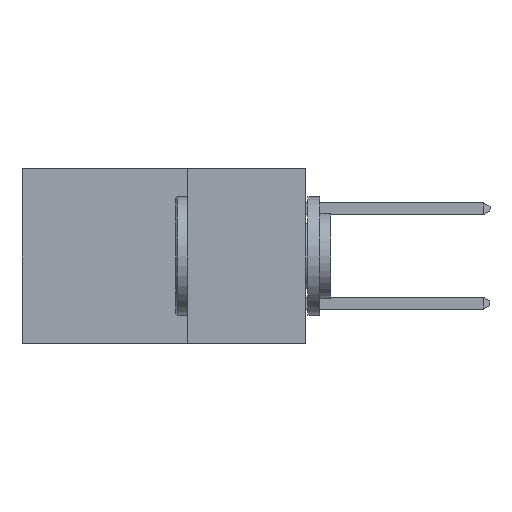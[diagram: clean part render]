
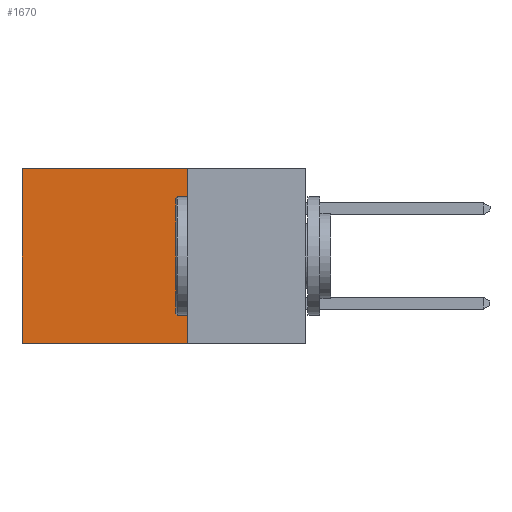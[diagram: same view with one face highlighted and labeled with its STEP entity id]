
A CAD part, left-side view. The second image highlights one B-rep face of the part: STEP entity #1670.
In plain terms, the highlighted planar face has unit normal (-1, 0, 0).
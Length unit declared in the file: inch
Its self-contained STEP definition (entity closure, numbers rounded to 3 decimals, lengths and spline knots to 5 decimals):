
#51 = CARTESIAN_POINT ( 'NONE',  ( 0.2615, 0.25, -0.37 ) ) ;
#232 = VERTEX_POINT ( 'NONE', #9290 ) ;
#253 = VERTEX_POINT ( 'NONE', #899 ) ;
#372 = ORIENTED_EDGE ( 'NONE', *, *, #7196, .F. ) ;
#837 = DIRECTION ( 'NONE',  ( 0., 0., -1. ) ) ;
#899 = CARTESIAN_POINT ( 'NONE',  ( 0.2615, 0.6, -0.37 ) ) ;
#1422 = CARTESIAN_POINT ( 'NONE',  ( 0.2615, 0.25, -0.37 ) ) ;
#1670 = ADVANCED_FACE ( 'NONE', ( #6097 ), #6054, .F. ) ;
#2181 = VECTOR ( 'NONE', #4646, 39.37008 ) ;
#2229 = CARTESIAN_POINT ( 'NONE',  ( 0.2615, 0.25, 0. ) ) ;
#2306 = DIRECTION ( 'NONE',  ( 0., 1., 0. ) ) ;
#3445 = VECTOR ( 'NONE', #7280, 39.37008 ) ;
#3839 = LINE ( 'NONE', #51, #5487 ) ;
#4253 = VERTEX_POINT ( 'NONE', #1422 ) ;
#4646 = DIRECTION ( 'NONE',  ( 0., 1., 0. ) ) ;
#4728 = ORIENTED_EDGE ( 'NONE', *, *, #7674, .F. ) ;
#5033 = VECTOR ( 'NONE', #2306, 39.37008 ) ;
#5055 = EDGE_LOOP ( 'NONE', ( #5706, #4728, #372, #9154 ) ) ;
#5148 = DIRECTION ( 'NONE',  ( 0., 0., -1. ) ) ;
#5487 = VECTOR ( 'NONE', #5148, 39.37008 ) ;
#5606 = EDGE_CURVE ( 'NONE', #8219, #253, #7429, .T. ) ;
#5706 = ORIENTED_EDGE ( 'NONE', *, *, #5606, .T. ) ;
#5981 = EDGE_CURVE ( 'NONE', #232, #8219, #8940, .T. ) ;
#6054 = PLANE ( 'NONE',  #9017 ) ;
#6056 = CARTESIAN_POINT ( 'NONE',  ( 0.2615, 0.25, -0.37 ) ) ;
#6097 = FACE_OUTER_BOUND ( 'NONE', #5055, .T. ) ;
#6509 = CARTESIAN_POINT ( 'NONE',  ( 0.2615, 0.6, -0.37 ) ) ;
#7196 = EDGE_CURVE ( 'NONE', #232, #4253, #3839, .T. ) ;
#7280 = DIRECTION ( 'NONE',  ( 0., 0., -1. ) ) ;
#7429 = LINE ( 'NONE', #6509, #3445 ) ;
#7554 = DIRECTION ( 'NONE',  ( 1., 0., 0. ) ) ;
#7674 = EDGE_CURVE ( 'NONE', #4253, #253, #9634, .T. ) ;
#8219 = VERTEX_POINT ( 'NONE', #9702 ) ;
#8940 = LINE ( 'NONE', #2229, #2181 ) ;
#9017 = AXIS2_PLACEMENT_3D ( 'NONE', #9026, #7554, #837 ) ;
#9026 = CARTESIAN_POINT ( 'NONE',  ( 0.2615, 0.25, -0.37 ) ) ;
#9154 = ORIENTED_EDGE ( 'NONE', *, *, #5981, .T. ) ;
#9290 = CARTESIAN_POINT ( 'NONE',  ( 0.2615, 0.25, 0. ) ) ;
#9634 = LINE ( 'NONE', #6056, #5033 ) ;
#9702 = CARTESIAN_POINT ( 'NONE',  ( 0.2615, 0.6, 0. ) ) ;
